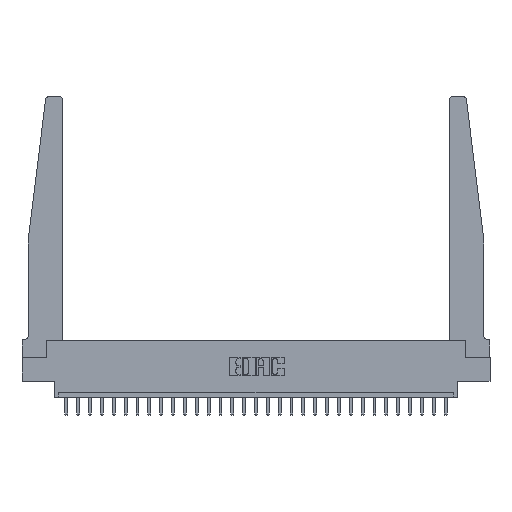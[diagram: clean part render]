
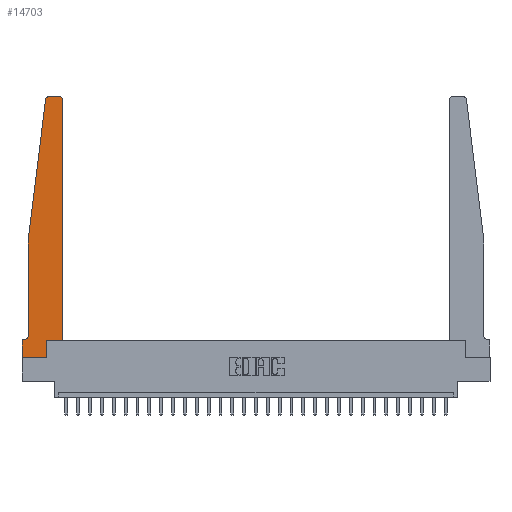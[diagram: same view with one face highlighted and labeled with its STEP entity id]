
A CAD part, top view. The second image highlights one B-rep face of the part: STEP entity #14703.
In plain terms, the highlighted planar face has unit normal (0, 0, 1).
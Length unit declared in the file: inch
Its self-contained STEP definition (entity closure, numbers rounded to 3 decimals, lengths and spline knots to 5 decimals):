
#226 = AXIS2_PLACEMENT_3D ( 'NONE', #24067, #22186, #11933 ) ;
#694 = CARTESIAN_POINT ( 'NONE',  ( 0.425, 0.18, 0.37 ) ) ;
#826 = EDGE_CURVE ( 'NONE', #14353, #13879, #17839, .T. ) ;
#917 = CARTESIAN_POINT ( 'NONE',  ( 0.065, 0.2375, 0.37 ) ) ;
#1045 = CARTESIAN_POINT ( 'NONE',  ( 0.065, 0.1875, 0.37 ) ) ;
#1403 = CIRCLE ( 'NONE', #25630, 0.05 ) ;
#2565 = VECTOR ( 'NONE', #21323, 39.37008 ) ;
#3301 = VERTEX_POINT ( 'NONE', #9629 ) ;
#3480 = CARTESIAN_POINT ( 'NONE',  ( 0., 0., 0.37 ) ) ;
#3601 = EDGE_CURVE ( 'NONE', #4746, #3301, #24738, .T. ) ;
#4105 = VERTEX_POINT ( 'NONE', #694 ) ;
#4257 = CARTESIAN_POINT ( 'NONE',  ( 0.425, 0.18, 0.37 ) ) ;
#4746 = VERTEX_POINT ( 'NONE', #18114 ) ;
#4944 = DIRECTION ( 'NONE',  ( -0.122, -0.992, 0. ) ) ;
#5762 = CARTESIAN_POINT ( 'NONE',  ( 0., 0., 0.37 ) ) ;
#5921 = CARTESIAN_POINT ( 'NONE',  ( 0., 0., 0.37 ) ) ;
#6267 = ORIENTED_EDGE ( 'NONE', *, *, #826, .T. ) ;
#6311 = CARTESIAN_POINT ( 'NONE',  ( 0.27653, 2.75, 0.37 ) ) ;
#6734 = VERTEX_POINT ( 'NONE', #11446 ) ;
#6753 = ORIENTED_EDGE ( 'NONE', *, *, #11895, .T. ) ;
#6769 = DIRECTION ( 'NONE',  ( -1., 0., 0. ) ) ;
#7147 = ORIENTED_EDGE ( 'NONE', *, *, #18548, .T. ) ;
#9275 = CARTESIAN_POINT ( 'NONE',  ( 0.065, 1.25, 0.37 ) ) ;
#9395 = VERTEX_POINT ( 'NONE', #6311 ) ;
#9495 = DIRECTION ( 'NONE',  ( -1., 0., 0. ) ) ;
#9506 = LINE ( 'NONE', #19664, #15294 ) ;
#9614 = DIRECTION ( 'NONE',  ( 0., 0., 1. ) ) ;
#9629 = CARTESIAN_POINT ( 'NONE',  ( 0.065, 1.25, 0.37 ) ) ;
#9750 = CARTESIAN_POINT ( 'NONE',  ( 0.2605, 0.18, 0.37 ) ) ;
#9925 = ORIENTED_EDGE ( 'NONE', *, *, #22042, .T. ) ;
#10415 = CIRCLE ( 'NONE', #18924, 0.03 ) ;
#10503 = DIRECTION ( 'NONE',  ( 0., 1., 0. ) ) ;
#10874 = CIRCLE ( 'NONE', #226, 0.03 ) ;
#11340 = ORIENTED_EDGE ( 'NONE', *, *, #16017, .T. ) ;
#11446 = CARTESIAN_POINT ( 'NONE',  ( 0.395, 2.75, 0.37 ) ) ;
#11895 = EDGE_CURVE ( 'NONE', #16572, #4105, #12568, .T. ) ;
#11913 = VECTOR ( 'NONE', #23479, 39.37008 ) ;
#11933 = DIRECTION ( 'NONE',  ( 1., 0., 0. ) ) ;
#12130 = DIRECTION ( 'NONE',  ( 1., 0., 0. ) ) ;
#12371 = EDGE_CURVE ( 'NONE', #4105, #24805, #16084, .T. ) ;
#12568 = LINE ( 'NONE', #4257, #11913 ) ;
#13267 = LINE ( 'NONE', #23531, #2565 ) ;
#13661 = CARTESIAN_POINT ( 'NONE',  ( 0.015, 0.1875, 0.37 ) ) ;
#13879 = VERTEX_POINT ( 'NONE', #22533 ) ;
#13926 = LINE ( 'NONE', #3480, #17196 ) ;
#14353 = VERTEX_POINT ( 'NONE', #5921 ) ;
#14451 = ORIENTED_EDGE ( 'NONE', *, *, #12371, .T. ) ;
#14528 = CARTESIAN_POINT ( 'NONE',  ( 0.425, 2.72, 0.37 ) ) ;
#14703 = ADVANCED_FACE ( 'NONE', ( #24277 ), #20361, .T. ) ;
#15002 = CARTESIAN_POINT ( 'NONE',  ( 0.425, 0.18, 0.37 ) ) ;
#15094 = EDGE_CURVE ( 'NONE', #24805, #6734, #10415, .T. ) ;
#15294 = VECTOR ( 'NONE', #17513, 39.37008 ) ;
#15673 = DIRECTION ( 'NONE',  ( 1., 0., 0. ) ) ;
#15835 = DIRECTION ( 'NONE',  ( 0., -1., 0. ) ) ;
#16017 = EDGE_CURVE ( 'NONE', #25785, #14353, #13926, .T. ) ;
#16049 = ORIENTED_EDGE ( 'NONE', *, *, #24042, .T. ) ;
#16084 = LINE ( 'NONE', #15002, #16410 ) ;
#16217 = CARTESIAN_POINT ( 'NONE',  ( 0., 0.1875, 0.37 ) ) ;
#16410 = VECTOR ( 'NONE', #10503, 39.37008 ) ;
#16572 = VERTEX_POINT ( 'NONE', #9750 ) ;
#17025 = DIRECTION ( 'NONE',  ( 1., 0., 0. ) ) ;
#17196 = VECTOR ( 'NONE', #15835, 39.37008 ) ;
#17513 = DIRECTION ( 'NONE',  ( -1., 0., 0. ) ) ;
#17684 = EDGE_CURVE ( 'NONE', #3301, #25191, #20984, .T. ) ;
#17839 = LINE ( 'NONE', #5762, #20716 ) ;
#18114 = CARTESIAN_POINT ( 'NONE',  ( 0.24675, 2.72367, 0.37 ) ) ;
#18548 = EDGE_CURVE ( 'NONE', #9395, #4746, #10874, .T. ) ;
#18924 = AXIS2_PLACEMENT_3D ( 'NONE', #19912, #9614, #15673 ) ;
#19067 = VECTOR ( 'NONE', #19659, 39.37008 ) ;
#19227 = DIRECTION ( 'NONE',  ( 0., 0., -1. ) ) ;
#19283 = EDGE_CURVE ( 'NONE', #25191, #20965, #1403, .T. ) ;
#19468 = EDGE_CURVE ( 'NONE', #6734, #9395, #9506, .T. ) ;
#19659 = DIRECTION ( 'NONE',  ( 0., -1., 0. ) ) ;
#19664 = CARTESIAN_POINT ( 'NONE',  ( 0.25, 2.75, 0.37 ) ) ;
#19912 = CARTESIAN_POINT ( 'NONE',  ( 0.395, 2.72, 0.37 ) ) ;
#20168 = CARTESIAN_POINT ( 'NONE',  ( 0.065, 1.25, 0.37 ) ) ;
#20361 = PLANE ( 'NONE',  #24897 ) ;
#20443 = DIRECTION ( 'NONE',  ( 0., 0., 1. ) ) ;
#20716 = VECTOR ( 'NONE', #17025, 39.37008 ) ;
#20890 = LINE ( 'NONE', #1045, #22811 ) ;
#20965 = VERTEX_POINT ( 'NONE', #13661 ) ;
#20984 = LINE ( 'NONE', #9275, #19067 ) ;
#21010 = EDGE_LOOP ( 'NONE', ( #26664, #7147, #21563, #24785, #24570, #16049, #11340, #6267, #9925, #6753, #14451, #23489 ) ) ;
#21282 = CARTESIAN_POINT ( 'NONE',  ( 0.015, 0.2375, 0.37 ) ) ;
#21323 = DIRECTION ( 'NONE',  ( 0., 1., 0. ) ) ;
#21563 = ORIENTED_EDGE ( 'NONE', *, *, #3601, .T. ) ;
#22042 = EDGE_CURVE ( 'NONE', #13879, #16572, #13267, .T. ) ;
#22186 = DIRECTION ( 'NONE',  ( 0., 0., 1. ) ) ;
#22497 = VECTOR ( 'NONE', #4944, 39.37008 ) ;
#22533 = CARTESIAN_POINT ( 'NONE',  ( 0.2605, 0., 0.37 ) ) ;
#22811 = VECTOR ( 'NONE', #9495, 39.37008 ) ;
#22873 = CARTESIAN_POINT ( 'NONE',  ( 0., 0.1875, 0.37 ) ) ;
#23479 = DIRECTION ( 'NONE',  ( 1., 0., 0. ) ) ;
#23489 = ORIENTED_EDGE ( 'NONE', *, *, #15094, .T. ) ;
#23531 = CARTESIAN_POINT ( 'NONE',  ( 0.2605, 0.18, 0.37 ) ) ;
#24042 = EDGE_CURVE ( 'NONE', #20965, #25785, #20890, .T. ) ;
#24067 = CARTESIAN_POINT ( 'NONE',  ( 0.27653, 2.72, 0.37 ) ) ;
#24277 = FACE_OUTER_BOUND ( 'NONE', #21010, .T. ) ;
#24570 = ORIENTED_EDGE ( 'NONE', *, *, #19283, .T. ) ;
#24738 = LINE ( 'NONE', #20168, #22497 ) ;
#24785 = ORIENTED_EDGE ( 'NONE', *, *, #17684, .T. ) ;
#24805 = VERTEX_POINT ( 'NONE', #14528 ) ;
#24897 = AXIS2_PLACEMENT_3D ( 'NONE', #16217, #20443, #12130 ) ;
#25191 = VERTEX_POINT ( 'NONE', #917 ) ;
#25630 = AXIS2_PLACEMENT_3D ( 'NONE', #21282, #19227, #6769 ) ;
#25785 = VERTEX_POINT ( 'NONE', #22873 ) ;
#26664 = ORIENTED_EDGE ( 'NONE', *, *, #19468, .T. ) ;
